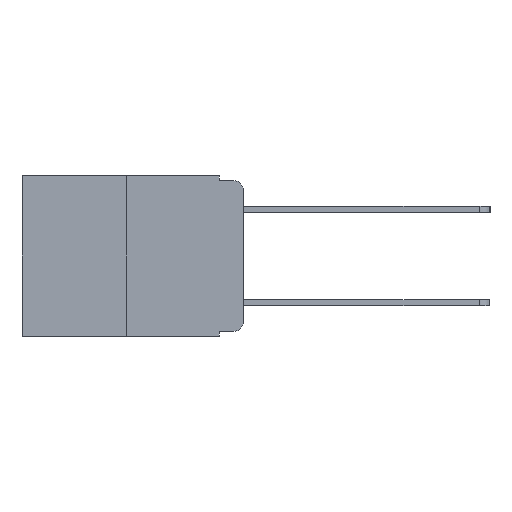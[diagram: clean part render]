
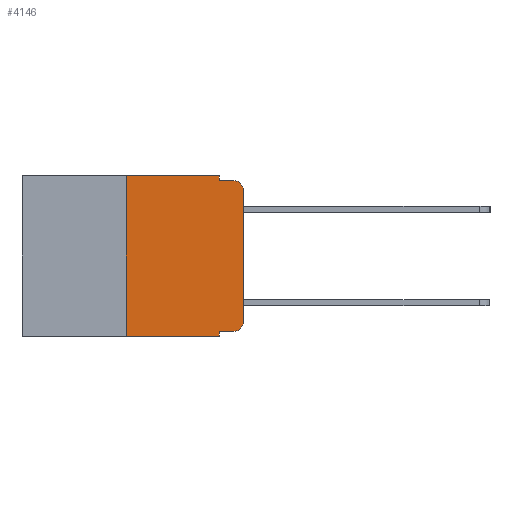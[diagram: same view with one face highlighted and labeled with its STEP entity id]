
A CAD part, left-side view. The second image highlights one B-rep face of the part: STEP entity #4146.
In plain terms, the highlighted planar face has unit normal (-1, 0, 0).
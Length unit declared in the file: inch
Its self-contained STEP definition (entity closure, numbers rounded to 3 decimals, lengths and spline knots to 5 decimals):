
#118 = LINE ( 'NONE', #768, #2729 ) ;
#197 = ORIENTED_EDGE ( 'NONE', *, *, #1714, .F. ) ;
#480 = VERTEX_POINT ( 'NONE', #11373 ) ;
#572 = DIRECTION ( 'NONE',  ( -1., 0., 0. ) ) ;
#707 = DIRECTION ( 'NONE',  ( 0., 0., -1. ) ) ;
#729 = CARTESIAN_POINT ( 'NONE',  ( 0., 0.02, -0.01 ) ) ;
#768 = CARTESIAN_POINT ( 'NONE',  ( 0., 0.473, 0. ) ) ;
#996 = DIRECTION ( 'NONE',  ( 0., 0., -1. ) ) ;
#1048 = VERTEX_POINT ( 'NONE', #9211 ) ;
#1147 = CARTESIAN_POINT ( 'NONE',  ( 0., 0.051, -0.333 ) ) ;
#1462 = PLANE ( 'NONE',  #6080 ) ;
#1714 = EDGE_CURVE ( 'NONE', #10234, #8047, #4349, .T. ) ;
#2050 = ORIENTED_EDGE ( 'NONE', *, *, #7751, .T. ) ;
#2125 = AXIS2_PLACEMENT_3D ( 'NONE', #6110, #572, #6967 ) ;
#2393 = EDGE_CURVE ( 'NONE', #11125, #7075, #3314, .T. ) ;
#2630 = EDGE_CURVE ( 'NONE', #11023, #6657, #11272, .T. ) ;
#2677 = DIRECTION ( 'NONE',  ( 0., -1., 0. ) ) ;
#2729 = VECTOR ( 'NONE', #2677, 39.37008 ) ;
#2753 = CARTESIAN_POINT ( 'NONE',  ( 0., 0.02, -0.333 ) ) ;
#2867 = VECTOR ( 'NONE', #10024, 39.37008 ) ;
#3080 = ORIENTED_EDGE ( 'NONE', *, *, #4159, .T. ) ;
#3137 = LINE ( 'NONE', #8742, #3446 ) ;
#3314 = CIRCLE ( 'NONE', #8590, 0.02 ) ;
#3373 = VERTEX_POINT ( 'NONE', #2753 ) ;
#3446 = VECTOR ( 'NONE', #3521, 39.37008 ) ;
#3521 = DIRECTION ( 'NONE',  ( 0., 0., -1. ) ) ;
#3670 = ORIENTED_EDGE ( 'NONE', *, *, #11006, .T. ) ;
#3673 = DIRECTION ( 'NONE',  ( 0., 0., 1. ) ) ;
#3680 = EDGE_CURVE ( 'NONE', #480, #5221, #3137, .T. ) ;
#3961 = CARTESIAN_POINT ( 'NONE',  ( 0., 0.051, -0.333 ) ) ;
#4053 = VECTOR ( 'NONE', #3673, 39.37008 ) ;
#4146 = ADVANCED_FACE ( 'NONE', ( #4150 ), #1462, .F. ) ;
#4150 = FACE_OUTER_BOUND ( 'NONE', #8676, .T. ) ;
#4159 = EDGE_CURVE ( 'NONE', #10234, #6657, #10993, .T. ) ;
#4349 = LINE ( 'NONE', #8198, #4053 ) ;
#4365 = CIRCLE ( 'NONE', #2125, 0.02 ) ;
#4651 = DIRECTION ( 'NONE',  ( 1., 0., 0. ) ) ;
#4762 = VECTOR ( 'NONE', #996, 39.37008 ) ;
#5214 = LINE ( 'NONE', #8624, #9526 ) ;
#5221 = VERTEX_POINT ( 'NONE', #11321 ) ;
#5233 = EDGE_CURVE ( 'NONE', #1048, #11125, #7103, .T. ) ;
#5287 = LINE ( 'NONE', #3961, #2867 ) ;
#6065 = DIRECTION ( 'NONE',  ( 0., -1., 0. ) ) ;
#6080 = AXIS2_PLACEMENT_3D ( 'NONE', #11113, #4651, #707 ) ;
#6110 = CARTESIAN_POINT ( 'NONE',  ( 0., 0.02, -0.313 ) ) ;
#6129 = DIRECTION ( 'NONE',  ( -1., 0., 0. ) ) ;
#6657 = VERTEX_POINT ( 'NONE', #9910 ) ;
#6967 = DIRECTION ( 'NONE',  ( 0., 0., -1. ) ) ;
#7075 = VERTEX_POINT ( 'NONE', #729 ) ;
#7103 = LINE ( 'NONE', #10242, #9144 ) ;
#7164 = CARTESIAN_POINT ( 'NONE',  ( 0., 0.02, -0.03 ) ) ;
#7751 = EDGE_CURVE ( 'NONE', #3373, #1048, #4365, .T. ) ;
#7908 = ORIENTED_EDGE ( 'NONE', *, *, #5233, .T. ) ;
#8047 = VERTEX_POINT ( 'NONE', #10660 ) ;
#8050 = ORIENTED_EDGE ( 'NONE', *, *, #2630, .F. ) ;
#8198 = CARTESIAN_POINT ( 'NONE',  ( 0., 0.25, 0. ) ) ;
#8337 = CARTESIAN_POINT ( 'NONE',  ( 0., 0.051, 0. ) ) ;
#8448 = ORIENTED_EDGE ( 'NONE', *, *, #2393, .T. ) ;
#8490 = VECTOR ( 'NONE', #11053, 39.37008 ) ;
#8539 = EDGE_CURVE ( 'NONE', #5221, #7075, #5214, .T. ) ;
#8590 = AXIS2_PLACEMENT_3D ( 'NONE', #7164, #6129, #11398 ) ;
#8624 = CARTESIAN_POINT ( 'NONE',  ( 0., 0.051, -0.01 ) ) ;
#8676 = EDGE_LOOP ( 'NONE', ( #7908, #8448, #8990, #11210, #11458, #197, #3080, #8050, #3670, #2050 ) ) ;
#8742 = CARTESIAN_POINT ( 'NONE',  ( 0., 0.051, 0. ) ) ;
#8908 = DIRECTION ( 'NONE',  ( 0., 0., 1. ) ) ;
#8990 = ORIENTED_EDGE ( 'NONE', *, *, #8539, .F. ) ;
#9144 = VECTOR ( 'NONE', #8908, 39.37008 ) ;
#9211 = CARTESIAN_POINT ( 'NONE',  ( 0., 0., -0.313 ) ) ;
#9391 = CARTESIAN_POINT ( 'NONE',  ( 0., 0.473, -0.343 ) ) ;
#9526 = VECTOR ( 'NONE', #6065, 39.37008 ) ;
#9647 = CARTESIAN_POINT ( 'NONE',  ( 0., 0.25, -0.343 ) ) ;
#9910 = CARTESIAN_POINT ( 'NONE',  ( 0., 0.051, -0.343 ) ) ;
#10024 = DIRECTION ( 'NONE',  ( 0., -1., 0. ) ) ;
#10234 = VERTEX_POINT ( 'NONE', #9647 ) ;
#10242 = CARTESIAN_POINT ( 'NONE',  ( 0., 0., 0. ) ) ;
#10660 = CARTESIAN_POINT ( 'NONE',  ( 0., 0.25, 0. ) ) ;
#10850 = EDGE_CURVE ( 'NONE', #8047, #480, #118, .T. ) ;
#10993 = LINE ( 'NONE', #9391, #8490 ) ;
#11006 = EDGE_CURVE ( 'NONE', #11023, #3373, #5287, .T. ) ;
#11023 = VERTEX_POINT ( 'NONE', #1147 ) ;
#11053 = DIRECTION ( 'NONE',  ( 0., -1., 0. ) ) ;
#11055 = CARTESIAN_POINT ( 'NONE',  ( 0., 0., -0.03 ) ) ;
#11113 = CARTESIAN_POINT ( 'NONE',  ( 0., 0.473, 0. ) ) ;
#11125 = VERTEX_POINT ( 'NONE', #11055 ) ;
#11210 = ORIENTED_EDGE ( 'NONE', *, *, #3680, .F. ) ;
#11272 = LINE ( 'NONE', #8337, #4762 ) ;
#11321 = CARTESIAN_POINT ( 'NONE',  ( 0., 0.051, -0.01 ) ) ;
#11373 = CARTESIAN_POINT ( 'NONE',  ( 0., 0.051, 0. ) ) ;
#11398 = DIRECTION ( 'NONE',  ( 0., 0., -1. ) ) ;
#11458 = ORIENTED_EDGE ( 'NONE', *, *, #10850, .F. ) ;
